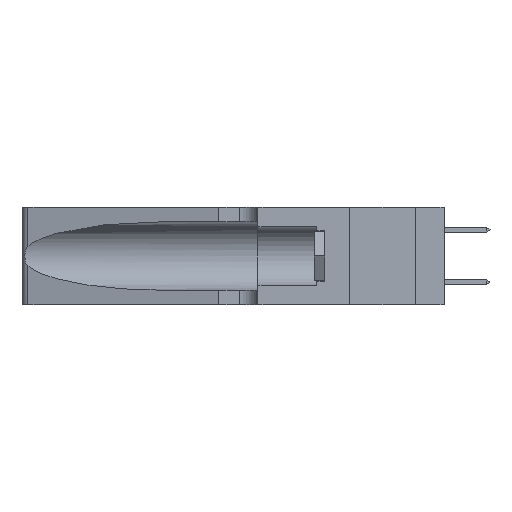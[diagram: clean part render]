
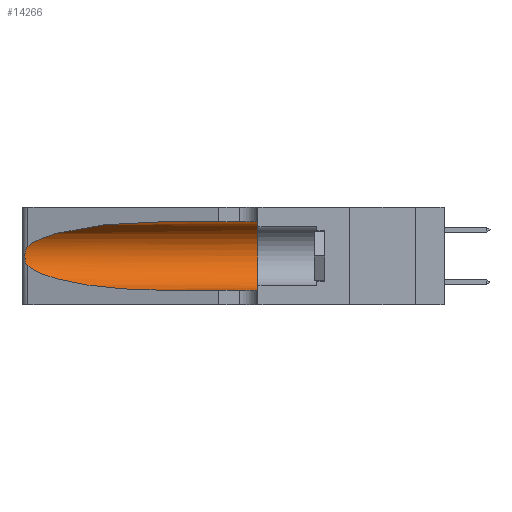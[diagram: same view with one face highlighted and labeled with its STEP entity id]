
A CAD part, left-side view. The second image highlights one B-rep face of the part: STEP entity #14266.
In plain terms, the highlighted cylindrical face has radius 3.308 mm (diameter 6.617 mm), a partial arc.
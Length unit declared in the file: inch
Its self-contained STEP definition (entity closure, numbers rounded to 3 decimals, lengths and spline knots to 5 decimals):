
#20 = EDGE_CURVE ( 'NONE', #10395, #16462, #17185, .T. ) ;
#127 = VERTEX_POINT ( 'NONE', #14939 ) ;
#638 = CARTESIAN_POINT ( 'NONE',  ( 0.25487, 1.22718, 0.22369 ) ) ;
#899 = DIRECTION ( 'NONE',  ( 0., -1., 0. ) ) ;
#917 =( BOUNDED_CURVE ( )  B_SPLINE_CURVE ( 3, ( #7913, #13514, #17685, #7851 ),
 .UNSPECIFIED., .F., .F. ) 
 B_SPLINE_CURVE_WITH_KNOTS ( ( 4, 4 ),
 ( 3.44316, 4.71239 ),
 .UNSPECIFIED. ) 
 CURVE ( )  GEOMETRIC_REPRESENTATION_ITEM ( )  RATIONAL_B_SPLINE_CURVE ( ( 1., 0.87, 0.87, 1. ) ) 
 REPRESENTATION_ITEM ( '' )  );
#939 = ORIENTED_EDGE ( 'NONE', *, *, #6620, .F. ) ;
#1543 = AXIS2_PLACEMENT_3D ( 'NONE', #14386, #13026, #17349 ) ;
#1622 = EDGE_CURVE ( 'NONE', #2081, #17737, #13461, .T. ) ;
#2081 = VERTEX_POINT ( 'NONE', #14241 ) ;
#2381 = ORIENTED_EDGE ( 'NONE', *, *, #3808, .T. ) ;
#2592 = CIRCLE ( 'NONE', #14894, 0.13025 ) ;
#2602 = CARTESIAN_POINT ( 'NONE',  ( 0.25487, 1.22718, 0.22369 ) ) ;
#3808 = EDGE_CURVE ( 'NONE', #12866, #10395, #9548, .T. ) ;
#4045 = CARTESIAN_POINT ( 'NONE',  ( 0.25639, 1.23184, 0.21858 ) ) ;
#4340 = CARTESIAN_POINT ( 'NONE',  ( 0.1305, 0.35, 0.185 ) ) ;
#4348 = CARTESIAN_POINT ( 'NONE',  ( 0.25639, 1.23186, 0.15144 ) ) ;
#4519 = CARTESIAN_POINT ( 'NONE',  ( 0.26075, 1.23896, 0.178 ) ) ;
#5060 = VECTOR ( 'NONE', #899, 39.37008 ) ;
#5468 = CARTESIAN_POINT ( 'NONE',  ( 0.25787, 1.23484, 0.2124 ) ) ;
#5847 = CARTESIAN_POINT ( 'NONE',  ( 0.25487, 1.22718, 0.14631 ) ) ;
#6042 = ORIENTED_EDGE ( 'NONE', *, *, #20, .T. ) ;
#6525 = CYLINDRICAL_SURFACE ( 'NONE', #1543, 0.13025 ) ;
#6620 = EDGE_CURVE ( 'NONE', #12866, #127, #10643, .T. ) ;
#7851 = CARTESIAN_POINT ( 'NONE',  ( 0.1305, 0.72297, 0.05475 ) ) ;
#7855 = FACE_OUTER_BOUND ( 'NONE', #16030, .T. ) ;
#7913 = CARTESIAN_POINT ( 'NONE',  ( 0.25487, 1.22718, 0.14631 ) ) ;
#7984 = ORIENTED_EDGE ( 'NONE', *, *, #17388, .T. ) ;
#8321 = CARTESIAN_POINT ( 'NONE',  ( 0.26018, 1.23835, 0.19895 ) ) ;
#8468 = CARTESIAN_POINT ( 'NONE',  ( 0.25487, 1.22718, 0.22369 ) ) ;
#8554 = CARTESIAN_POINT ( 'NONE',  ( 0.1305, 0.72297, 0.31525 ) ) ;
#8647 = CARTESIAN_POINT ( 'NONE',  ( 0.25856, 1.23593, 0.16098 ) ) ;
#8885 = ORIENTED_EDGE ( 'NONE', *, *, #1622, .T. ) ;
#9139 = CARTESIAN_POINT ( 'NONE',  ( 0.1305, 1.61858, 0.05475 ) ) ;
#9548 =( BOUNDED_CURVE ( )  B_SPLINE_CURVE ( 3, ( #15491, #16944, #15553, #8468 ),
 .UNSPECIFIED., .F., .F. ) 
 B_SPLINE_CURVE_WITH_KNOTS ( ( 4, 4 ),
 ( 1.5708, 2.84003 ),
 .UNSPECIFIED. ) 
 CURVE ( )  GEOMETRIC_REPRESENTATION_ITEM ( )  RATIONAL_B_SPLINE_CURVE ( ( 1., 0.87, 0.87, 1. ) ) 
 REPRESENTATION_ITEM ( '' )  );
#10258 = CARTESIAN_POINT ( 'NONE',  ( 0.25555, 1.22993, 0.14849 ) ) ;
#10395 = VERTEX_POINT ( 'NONE', #638 ) ;
#10572 = DIRECTION ( 'NONE',  ( 0., 0., 1. ) ) ;
#10643 = LINE ( 'NONE', #12199, #5060 ) ;
#11759 = EDGE_CURVE ( 'NONE', #127, #17737, #2592, .T. ) ;
#11832 = DIRECTION ( 'NONE',  ( 0., 1., 0. ) ) ;
#12199 = CARTESIAN_POINT ( 'NONE',  ( 0.1305, 1.61858, 0.31525 ) ) ;
#12274 = ORIENTED_EDGE ( 'NONE', *, *, #11759, .F. ) ;
#12789 = CARTESIAN_POINT ( 'NONE',  ( 0.25487, 1.22718, 0.14631 ) ) ;
#12866 = VERTEX_POINT ( 'NONE', #8554 ) ;
#13026 = DIRECTION ( 'NONE',  ( 0., -1., 0. ) ) ;
#13409 = DIRECTION ( 'NONE',  ( 0., -1., 0. ) ) ;
#13461 = LINE ( 'NONE', #9139, #14348 ) ;
#13514 = CARTESIAN_POINT ( 'NONE',  ( 0.2373, 1.15595, 0.08982 ) ) ;
#14241 = CARTESIAN_POINT ( 'NONE',  ( 0.1305, 0.72297, 0.05475 ) ) ;
#14266 = ADVANCED_FACE ( 'NONE', ( #7855 ), #6525, .F. ) ;
#14348 = VECTOR ( 'NONE', #13409, 39.37008 ) ;
#14386 = CARTESIAN_POINT ( 'NONE',  ( 0.1305, 1.61858, 0.185 ) ) ;
#14894 = AXIS2_PLACEMENT_3D ( 'NONE', #4340, #11832, #10572 ) ;
#14939 = CARTESIAN_POINT ( 'NONE',  ( 0.1305, 0.35, 0.31525 ) ) ;
#15414 = CARTESIAN_POINT ( 'NONE',  ( 0.25854, 1.2359, 0.20912 ) ) ;
#15491 = CARTESIAN_POINT ( 'NONE',  ( 0.1305, 0.72297, 0.31525 ) ) ;
#15553 = CARTESIAN_POINT ( 'NONE',  ( 0.2373, 1.15595, 0.28018 ) ) ;
#15835 = CARTESIAN_POINT ( 'NONE',  ( 0.26017, 1.23833, 0.17102 ) ) ;
#16030 = EDGE_LOOP ( 'NONE', ( #2381, #6042, #7984, #8885, #12274, #939 ) ) ;
#16462 = VERTEX_POINT ( 'NONE', #5847 ) ;
#16809 = CARTESIAN_POINT ( 'NONE',  ( 0.25555, 1.22994, 0.2215 ) ) ;
#16944 = CARTESIAN_POINT ( 'NONE',  ( 0.18966, 0.96281, 0.31525 ) ) ;
#17185 = B_SPLINE_CURVE_WITH_KNOTS ( 'NONE', 3,
 ( #2602, #16809, #4045, #5468, #15414, #8321, #18281, #4519, #15835, #8647, #17227, #4348, #10258, #12789 ),
 .UNSPECIFIED., .F., .F.,
 ( 4, 2, 2, 2, 2, 2, 4 ),
 ( 0., 0.00027, 0.00053, 0.00107, 0.0016, 0.00187, 0.00214 ),
 .UNSPECIFIED. ) ;
#17197 = CARTESIAN_POINT ( 'NONE',  ( 0.1305, 0.35, 0.05475 ) ) ;
#17227 = CARTESIAN_POINT ( 'NONE',  ( 0.25789, 1.23486, 0.15765 ) ) ;
#17349 = DIRECTION ( 'NONE',  ( 0., 0., -1. ) ) ;
#17388 = EDGE_CURVE ( 'NONE', #16462, #2081, #917, .T. ) ;
#17685 = CARTESIAN_POINT ( 'NONE',  ( 0.18966, 0.96281, 0.05475 ) ) ;
#17737 = VERTEX_POINT ( 'NONE', #17197 ) ;
#18281 = CARTESIAN_POINT ( 'NONE',  ( 0.26075, 1.23896, 0.19203 ) ) ;
